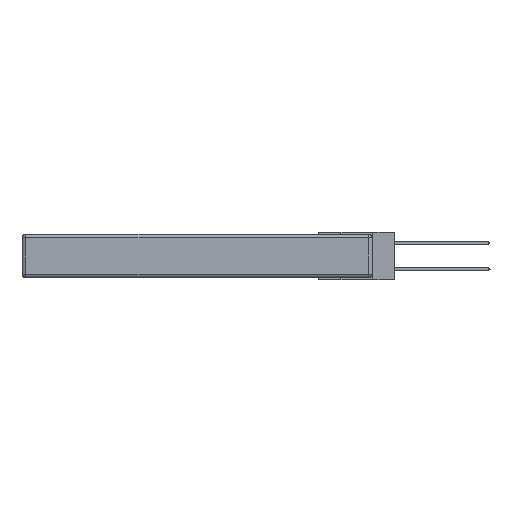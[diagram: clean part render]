
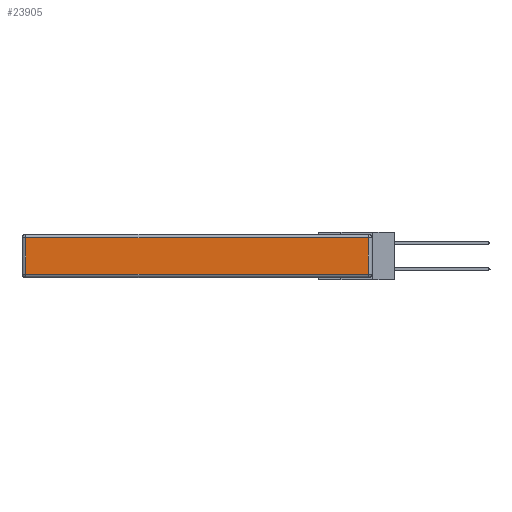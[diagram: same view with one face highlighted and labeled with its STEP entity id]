
A CAD part, left-side view. The second image highlights one B-rep face of the part: STEP entity #23905.
In plain terms, the highlighted planar face has unit normal (-1, 0, 0).
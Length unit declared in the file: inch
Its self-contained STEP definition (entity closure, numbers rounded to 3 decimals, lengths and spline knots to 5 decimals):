
#1812 = VERTEX_POINT ( 'NONE', #3999 ) ;
#1970 = AXIS2_PLACEMENT_3D ( 'NONE', #4178, #21550, #13106 ) ;
#2260 = PLANE ( 'NONE',  #1970 ) ;
#2592 = VERTEX_POINT ( 'NONE', #21619 ) ;
#2693 = VERTEX_POINT ( 'NONE', #22668 ) ;
#3212 = DIRECTION ( 'NONE',  ( 0., 0., -1. ) ) ;
#3820 = DIRECTION ( 'NONE',  ( 0., 0., 1. ) ) ;
#3999 = CARTESIAN_POINT ( 'NONE',  ( 0., 2.72, -0.313 ) ) ;
#4178 = CARTESIAN_POINT ( 'NONE',  ( 0., 0., -0.343 ) ) ;
#4998 = EDGE_CURVE ( 'NONE', #6336, #1812, #15821, .T. ) ;
#6336 = VERTEX_POINT ( 'NONE', #24844 ) ;
#7823 = FACE_OUTER_BOUND ( 'NONE', #27051, .T. ) ;
#7829 = EDGE_CURVE ( 'NONE', #2693, #2592, #11921, .T. ) ;
#9548 = VECTOR ( 'NONE', #3820, 39.37008 ) ;
#9945 = CARTESIAN_POINT ( 'NONE',  ( 0., 2.72, -0.343 ) ) ;
#11806 = CARTESIAN_POINT ( 'NONE',  ( 0., 2.75, -0.03 ) ) ;
#11921 = LINE ( 'NONE', #27947, #9548 ) ;
#13106 = DIRECTION ( 'NONE',  ( 0., 0., 1. ) ) ;
#14133 = VECTOR ( 'NONE', #3212, 39.37008 ) ;
#15821 = LINE ( 'NONE', #9945, #14133 ) ;
#17110 = EDGE_CURVE ( 'NONE', #1812, #2693, #21284, .T. ) ;
#19418 = LINE ( 'NONE', #11806, #25947 ) ;
#20325 = ORIENTED_EDGE ( 'NONE', *, *, #17110, .T. ) ;
#20398 = EDGE_CURVE ( 'NONE', #2592, #6336, #19418, .T. ) ;
#21284 = LINE ( 'NONE', #28075, #28150 ) ;
#21392 = ORIENTED_EDGE ( 'NONE', *, *, #7829, .T. ) ;
#21550 = DIRECTION ( 'NONE',  ( -1., 0., 0. ) ) ;
#21619 = CARTESIAN_POINT ( 'NONE',  ( 0., 0.03, -0.03 ) ) ;
#22668 = CARTESIAN_POINT ( 'NONE',  ( 0., 0.03, -0.313 ) ) ;
#23905 = ADVANCED_FACE ( 'NONE', ( #7823 ), #2260, .T. ) ;
#24844 = CARTESIAN_POINT ( 'NONE',  ( 0., 2.72, -0.03 ) ) ;
#25947 = VECTOR ( 'NONE', #27086, 39.37008 ) ;
#26511 = ORIENTED_EDGE ( 'NONE', *, *, #20398, .T. ) ;
#27051 = EDGE_LOOP ( 'NONE', ( #20325, #21392, #26511, #28104 ) ) ;
#27086 = DIRECTION ( 'NONE',  ( 0., 1., 0. ) ) ;
#27771 = DIRECTION ( 'NONE',  ( 0., -1., 0. ) ) ;
#27947 = CARTESIAN_POINT ( 'NONE',  ( 0., 0.03, -0.343 ) ) ;
#28075 = CARTESIAN_POINT ( 'NONE',  ( 0., 0., -0.313 ) ) ;
#28104 = ORIENTED_EDGE ( 'NONE', *, *, #4998, .T. ) ;
#28150 = VECTOR ( 'NONE', #27771, 39.37008 ) ;
